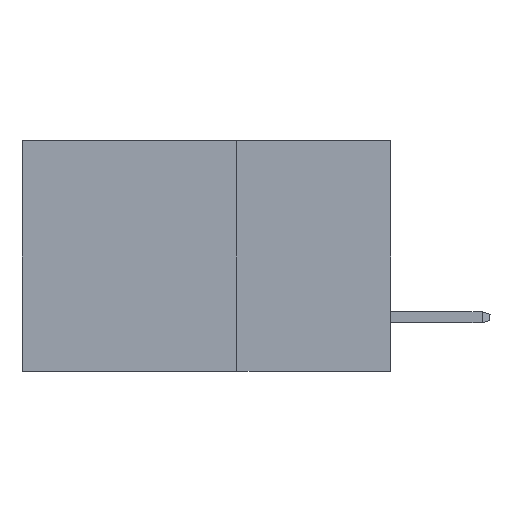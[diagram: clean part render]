
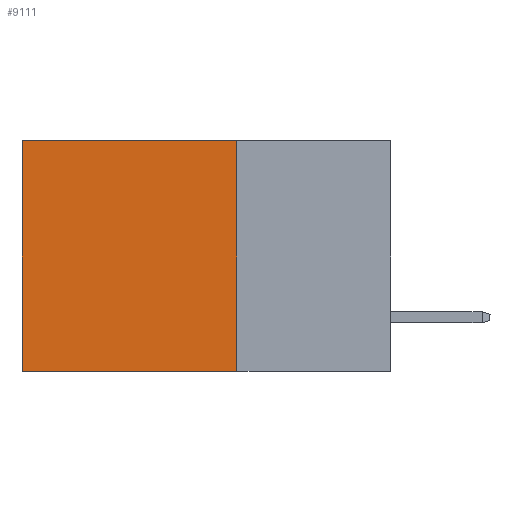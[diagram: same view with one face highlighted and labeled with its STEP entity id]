
A CAD part, left-side view. The second image highlights one B-rep face of the part: STEP entity #9111.
In plain terms, the highlighted planar face has unit normal (-1, 0, 0).
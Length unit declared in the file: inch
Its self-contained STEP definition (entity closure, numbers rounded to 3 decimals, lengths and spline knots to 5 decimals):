
#3388 = LINE ( 'NONE', #9269, #5661 ) ;
#4078 = CARTESIAN_POINT ( 'NONE',  ( 0.2875, 0.25, -0.375 ) ) ;
#4220 = CARTESIAN_POINT ( 'NONE',  ( 0.2875, 0.25, 0. ) ) ;
#4583 = EDGE_CURVE ( 'NONE', #11067, #6378, #19997, .T. ) ;
#4708 = EDGE_CURVE ( 'NONE', #6319, #6378, #5532, .T. ) ;
#4945 = ORIENTED_EDGE ( 'NONE', *, *, #11494, .T. ) ;
#5026 = CARTESIAN_POINT ( 'NONE',  ( 0.2875, 0.6, -0.375 ) ) ;
#5053 = LINE ( 'NONE', #4078, #16209 ) ;
#5269 = CARTESIAN_POINT ( 'NONE',  ( 0.2875, 0.25, -0.375 ) ) ;
#5532 = LINE ( 'NONE', #5026, #15184 ) ;
#5661 = VECTOR ( 'NONE', #9194, 39.37008 ) ;
#6092 = CARTESIAN_POINT ( 'NONE',  ( 0.2875, 0.25, -0.375 ) ) ;
#6319 = VERTEX_POINT ( 'NONE', #10009 ) ;
#6378 = VERTEX_POINT ( 'NONE', #17905 ) ;
#6818 = DIRECTION ( 'NONE',  ( 0., 0., -1. ) ) ;
#7938 = ORIENTED_EDGE ( 'NONE', *, *, #4583, .F. ) ;
#8253 = PLANE ( 'NONE',  #9735 ) ;
#9111 = ADVANCED_FACE ( 'NONE', ( #11670 ), #8253, .F. ) ;
#9194 = DIRECTION ( 'NONE',  ( 0., 1., 0. ) ) ;
#9269 = CARTESIAN_POINT ( 'NONE',  ( 0.2875, 0.25, 0. ) ) ;
#9588 = DIRECTION ( 'NONE',  ( 0., 1., 0. ) ) ;
#9735 = AXIS2_PLACEMENT_3D ( 'NONE', #5269, #18228, #6818 ) ;
#9875 = DIRECTION ( 'NONE',  ( 0., 0., -1. ) ) ;
#10009 = CARTESIAN_POINT ( 'NONE',  ( 0.2875, 0.6, 0. ) ) ;
#10597 = ORIENTED_EDGE ( 'NONE', *, *, #4708, .T. ) ;
#11067 = VERTEX_POINT ( 'NONE', #17488 ) ;
#11494 = EDGE_CURVE ( 'NONE', #13065, #6319, #3388, .T. ) ;
#11670 = FACE_OUTER_BOUND ( 'NONE', #19841, .T. ) ;
#13065 = VERTEX_POINT ( 'NONE', #4220 ) ;
#14155 = VECTOR ( 'NONE', #9588, 39.37008 ) ;
#15184 = VECTOR ( 'NONE', #9875, 39.37008 ) ;
#16209 = VECTOR ( 'NONE', #18663, 39.37008 ) ;
#17488 = CARTESIAN_POINT ( 'NONE',  ( 0.2875, 0.25, -0.375 ) ) ;
#17769 = ORIENTED_EDGE ( 'NONE', *, *, #18967, .F. ) ;
#17905 = CARTESIAN_POINT ( 'NONE',  ( 0.2875, 0.6, -0.375 ) ) ;
#18228 = DIRECTION ( 'NONE',  ( 1., 0., 0. ) ) ;
#18663 = DIRECTION ( 'NONE',  ( 0., 0., -1. ) ) ;
#18967 = EDGE_CURVE ( 'NONE', #13065, #11067, #5053, .T. ) ;
#19841 = EDGE_LOOP ( 'NONE', ( #10597, #7938, #17769, #4945 ) ) ;
#19997 = LINE ( 'NONE', #6092, #14155 ) ;
